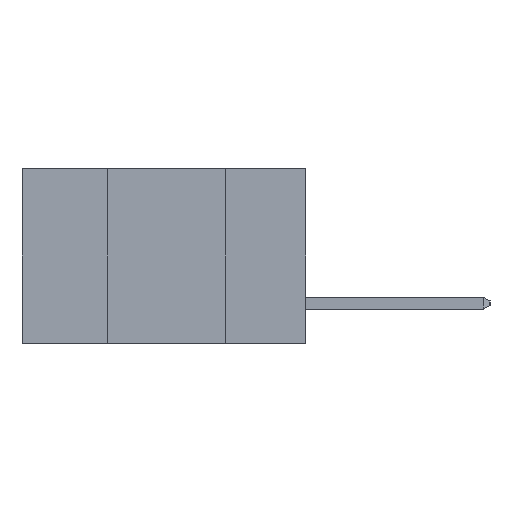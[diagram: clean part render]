
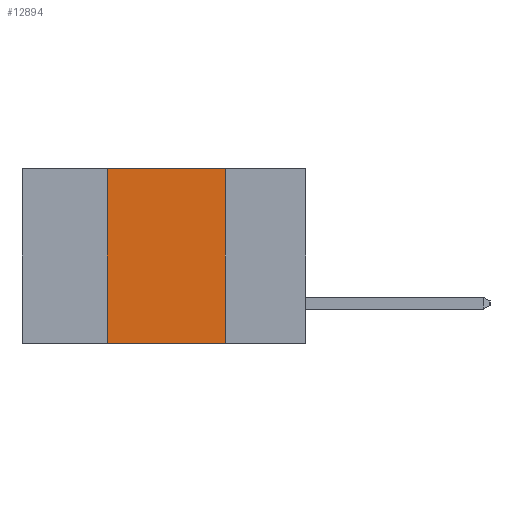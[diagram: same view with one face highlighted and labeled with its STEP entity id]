
A CAD part, left-side view. The second image highlights one B-rep face of the part: STEP entity #12894.
In plain terms, the highlighted planar face has unit normal (-1, 0, 0).
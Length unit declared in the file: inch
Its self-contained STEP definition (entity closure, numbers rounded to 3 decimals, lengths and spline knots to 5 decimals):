
#763 = CARTESIAN_POINT ( 'NONE',  ( 0., 0.17, -0.37 ) ) ;
#1814 = VERTEX_POINT ( 'NONE', #3707 ) ;
#1859 = EDGE_CURVE ( 'NONE', #1863, #2893, #10487, .T. ) ;
#1863 = VERTEX_POINT ( 'NONE', #11774 ) ;
#2150 = EDGE_LOOP ( 'NONE', ( #10297, #7593, #7107, #5489 ) ) ;
#2190 = CARTESIAN_POINT ( 'NONE',  ( 0., 0.42, 0. ) ) ;
#2775 = DIRECTION ( 'NONE',  ( 0., 0., -1. ) ) ;
#2893 = VERTEX_POINT ( 'NONE', #763 ) ;
#3081 = VECTOR ( 'NONE', #5632, 39.37008 ) ;
#3707 = CARTESIAN_POINT ( 'NONE',  ( 0., 0.42, -0.37 ) ) ;
#5489 = ORIENTED_EDGE ( 'NONE', *, *, #14431, .T. ) ;
#5632 = DIRECTION ( 'NONE',  ( 0., -1., 0. ) ) ;
#6782 = LINE ( 'NONE', #17251, #3081 ) ;
#6875 = DIRECTION ( 'NONE',  ( 0., 0., 1. ) ) ;
#6955 = VECTOR ( 'NONE', #13206, 39.37008 ) ;
#7107 = ORIENTED_EDGE ( 'NONE', *, *, #7447, .F. ) ;
#7154 = CARTESIAN_POINT ( 'NONE',  ( 0., 0.42, 0. ) ) ;
#7447 = EDGE_CURVE ( 'NONE', #1814, #15584, #16186, .T. ) ;
#7593 = ORIENTED_EDGE ( 'NONE', *, *, #14637, .F. ) ;
#9358 = VECTOR ( 'NONE', #6875, 39.37008 ) ;
#10151 = VECTOR ( 'NONE', #11473, 39.37008 ) ;
#10297 = ORIENTED_EDGE ( 'NONE', *, *, #1859, .F. ) ;
#10487 = LINE ( 'NONE', #11585, #6955 ) ;
#10897 = DIRECTION ( 'NONE',  ( 1., 0., 0. ) ) ;
#11473 = DIRECTION ( 'NONE',  ( 0., -1., 0. ) ) ;
#11585 = CARTESIAN_POINT ( 'NONE',  ( 0., 0.17, 0. ) ) ;
#11774 = CARTESIAN_POINT ( 'NONE',  ( 0., 0.17, 0. ) ) ;
#12894 = ADVANCED_FACE ( 'NONE', ( #12982 ), #13441, .F. ) ;
#12982 = FACE_OUTER_BOUND ( 'NONE', #2150, .T. ) ;
#13206 = DIRECTION ( 'NONE',  ( 0., 0., -1. ) ) ;
#13441 = PLANE ( 'NONE',  #17106 ) ;
#13567 = LINE ( 'NONE', #16539, #10151 ) ;
#14431 = EDGE_CURVE ( 'NONE', #1814, #2893, #13567, .T. ) ;
#14637 = EDGE_CURVE ( 'NONE', #15584, #1863, #6782, .T. ) ;
#15584 = VERTEX_POINT ( 'NONE', #2190 ) ;
#15998 = CARTESIAN_POINT ( 'NONE',  ( 0., 0.6, 0. ) ) ;
#16186 = LINE ( 'NONE', #7154, #9358 ) ;
#16539 = CARTESIAN_POINT ( 'NONE',  ( 0., 0.6, -0.37 ) ) ;
#17106 = AXIS2_PLACEMENT_3D ( 'NONE', #15998, #10897, #2775 ) ;
#17251 = CARTESIAN_POINT ( 'NONE',  ( 0., 0.6, 0. ) ) ;
